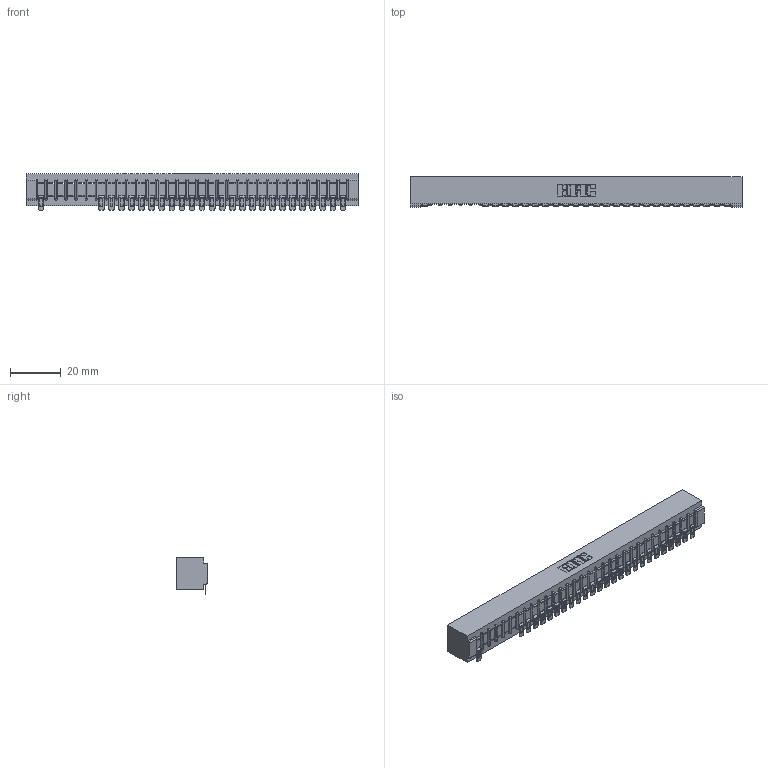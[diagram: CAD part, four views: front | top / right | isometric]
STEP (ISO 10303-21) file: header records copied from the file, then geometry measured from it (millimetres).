
FILE_DESCRIPTION (( 'STEP AP203' ), '1' );
FILE_NAME ('357-031-554-101.STEP', '2018-08-09T22:51:05', ( '' ), ( '' ), 'SwSTEP 2.0', 'SolidWorks 2016', '' );
FILE_SCHEMA (( 'CONFIG_CONTROL_DESIGN' ));
Length unit declared in the file: inch
Products named in the file (3): 307-290-002_554; 357-031-554-101; 307 Part_No Mounting Lugs
Assembly tree (27 placements, depth 2):
  357-031-554-101
    307 Part_No Mounting Lugs
    307-290-002_554  x26
Bounding box: 130.71 x 12.01 x 14.52 mm (x, y, z)
Volume: 14327.9 mm3; surface area: 17297.5 mm2
Topology: 27 solids, 27 shells, 2348 faces, 7197 edges, 4710 vertices
Faces by surface type: plane 1322, cylinder 962, sphere 64
Entity records: 28459 total; most frequent: CARTESIAN_POINT 4821, ORIENTED_EDGE 4816, DIRECTION 4688, EDGE_CURVE 2408, VECTOR 1834, LINE 1834, VERTEX_POINT 1560, AXIS2_PLACEMENT_3D 1427
